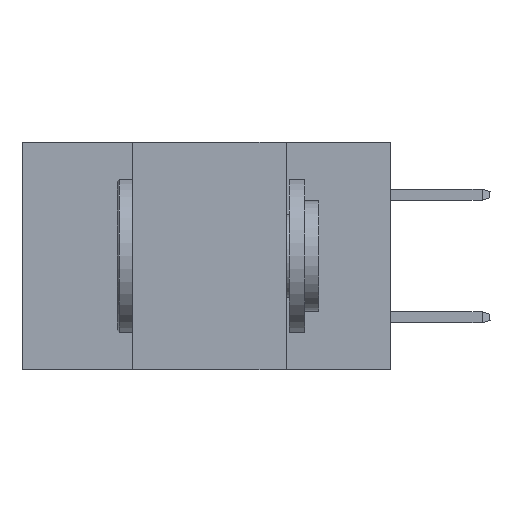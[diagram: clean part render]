
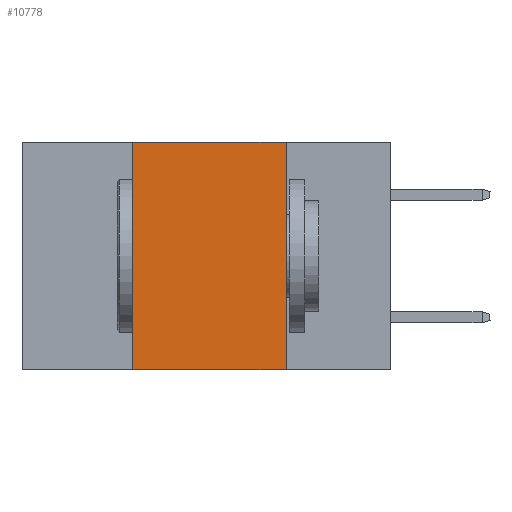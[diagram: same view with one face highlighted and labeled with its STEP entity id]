
A CAD part, left-side view. The second image highlights one B-rep face of the part: STEP entity #10778.
In plain terms, the highlighted planar face has unit normal (-1, 0, 0).
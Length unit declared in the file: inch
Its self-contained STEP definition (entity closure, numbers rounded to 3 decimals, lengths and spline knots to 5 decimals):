
#112 = VECTOR ( 'NONE', #10113, 39.37008 ) ;
#166 = AXIS2_PLACEMENT_3D ( 'NONE', #6187, #2805, #8640 ) ;
#191 = FACE_OUTER_BOUND ( 'NONE', #4363, .T. ) ;
#724 = LINE ( 'NONE', #969, #5259 ) ;
#809 = PLANE ( 'NONE',  #166 ) ;
#969 = CARTESIAN_POINT ( 'NONE',  ( 0., 0.17, 0. ) ) ;
#1616 = VERTEX_POINT ( 'NONE', #8180 ) ;
#2554 = VERTEX_POINT ( 'NONE', #6818 ) ;
#2708 = ORIENTED_EDGE ( 'NONE', *, *, #10991, .F. ) ;
#2805 = DIRECTION ( 'NONE',  ( 1., 0., 0. ) ) ;
#3182 = DIRECTION ( 'NONE',  ( 0., -1., 0. ) ) ;
#3680 = EDGE_CURVE ( 'NONE', #8388, #2554, #724, .T. ) ;
#3687 = CARTESIAN_POINT ( 'NONE',  ( 0., 0.17, 0. ) ) ;
#4363 = EDGE_LOOP ( 'NONE', ( #6947, #2708, #7454, #9634 ) ) ;
#4768 = LINE ( 'NONE', #10156, #112 ) ;
#4789 = CARTESIAN_POINT ( 'NONE',  ( 0., 0.42, 0. ) ) ;
#5259 = VECTOR ( 'NONE', #7670, 39.37008 ) ;
#5339 = DIRECTION ( 'NONE',  ( 0., 0., 1. ) ) ;
#6187 = CARTESIAN_POINT ( 'NONE',  ( 0., 0.6, 0. ) ) ;
#6335 = VECTOR ( 'NONE', #5339, 39.37008 ) ;
#6818 = CARTESIAN_POINT ( 'NONE',  ( 0., 0.17, -0.37 ) ) ;
#6882 = EDGE_CURVE ( 'NONE', #1616, #7911, #8492, .T. ) ;
#6947 = ORIENTED_EDGE ( 'NONE', *, *, #3680, .F. ) ;
#7097 = EDGE_CURVE ( 'NONE', #1616, #2554, #4768, .T. ) ;
#7454 = ORIENTED_EDGE ( 'NONE', *, *, #6882, .F. ) ;
#7670 = DIRECTION ( 'NONE',  ( 0., 0., -1. ) ) ;
#7911 = VERTEX_POINT ( 'NONE', #4789 ) ;
#8154 = CARTESIAN_POINT ( 'NONE',  ( 0., 0.6, 0. ) ) ;
#8180 = CARTESIAN_POINT ( 'NONE',  ( 0., 0.42, -0.37 ) ) ;
#8388 = VERTEX_POINT ( 'NONE', #3687 ) ;
#8492 = LINE ( 'NONE', #10619, #6335 ) ;
#8541 = VECTOR ( 'NONE', #3182, 39.37008 ) ;
#8640 = DIRECTION ( 'NONE',  ( 0., 0., -1. ) ) ;
#9634 = ORIENTED_EDGE ( 'NONE', *, *, #7097, .T. ) ;
#10113 = DIRECTION ( 'NONE',  ( 0., -1., 0. ) ) ;
#10156 = CARTESIAN_POINT ( 'NONE',  ( 0., 0.6, -0.37 ) ) ;
#10448 = LINE ( 'NONE', #8154, #8541 ) ;
#10619 = CARTESIAN_POINT ( 'NONE',  ( 0., 0.42, 0. ) ) ;
#10778 = ADVANCED_FACE ( 'NONE', ( #191 ), #809, .F. ) ;
#10991 = EDGE_CURVE ( 'NONE', #7911, #8388, #10448, .T. ) ;
